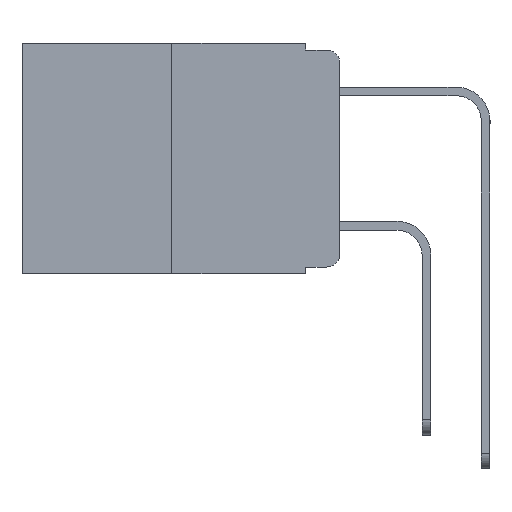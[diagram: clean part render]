
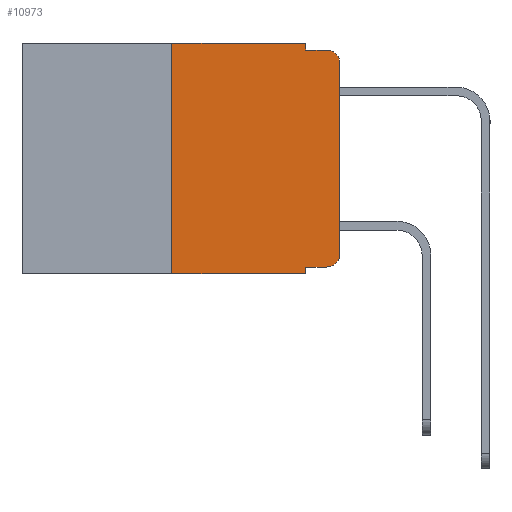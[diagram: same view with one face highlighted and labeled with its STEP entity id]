
A CAD part, left-side view. The second image highlights one B-rep face of the part: STEP entity #10973.
In plain terms, the highlighted planar face has unit normal (-1, 0, 0).
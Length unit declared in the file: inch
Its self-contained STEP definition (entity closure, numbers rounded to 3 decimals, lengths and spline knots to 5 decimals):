
#121 = CARTESIAN_POINT ( 'NONE',  ( 0., 0.25, 0. ) ) ;
#300 = CARTESIAN_POINT ( 'NONE',  ( 0., 0.02, -0.313 ) ) ;
#713 = VECTOR ( 'NONE', #7332, 39.37008 ) ;
#1309 = VECTOR ( 'NONE', #12320, 39.37008 ) ;
#1581 = VERTEX_POINT ( 'NONE', #13843 ) ;
#1685 = CARTESIAN_POINT ( 'NONE',  ( 0., 0.473, -0.343 ) ) ;
#1734 = CARTESIAN_POINT ( 'NONE',  ( 0., 0.473, 0. ) ) ;
#1775 = CARTESIAN_POINT ( 'NONE',  ( 0., 0.051, 0. ) ) ;
#1842 = VECTOR ( 'NONE', #8486, 39.37008 ) ;
#1939 = EDGE_CURVE ( 'NONE', #2662, #12928, #4827, .T. ) ;
#1991 = EDGE_CURVE ( 'NONE', #5677, #5388, #7577, .T. ) ;
#2223 = DIRECTION ( 'NONE',  ( 0., 0., -1. ) ) ;
#2230 = DIRECTION ( 'NONE',  ( -1., 0., 0. ) ) ;
#2281 = VECTOR ( 'NONE', #14022, 39.37008 ) ;
#2423 = AXIS2_PLACEMENT_3D ( 'NONE', #7791, #16998, #9151 ) ;
#2506 = EDGE_CURVE ( 'NONE', #15991, #2662, #7138, .T. ) ;
#2662 = VERTEX_POINT ( 'NONE', #10346 ) ;
#2680 = CARTESIAN_POINT ( 'NONE',  ( 0., 0.051, 0. ) ) ;
#2970 = LINE ( 'NONE', #5135, #10145 ) ;
#3116 = CARTESIAN_POINT ( 'NONE',  ( 0., 0.473, 0. ) ) ;
#3164 = DIRECTION ( 'NONE',  ( 0., 0., -1. ) ) ;
#3512 = ORIENTED_EDGE ( 'NONE', *, *, #13549, .T. ) ;
#4328 = CARTESIAN_POINT ( 'NONE',  ( 0., 0.051, -0.333 ) ) ;
#4356 = EDGE_LOOP ( 'NONE', ( #6258, #3512, #14533, #4379, #8795, #9228, #12717, #9637, #6898, #10875 ) ) ;
#4379 = ORIENTED_EDGE ( 'NONE', *, *, #13575, .F. ) ;
#4827 = LINE ( 'NONE', #7327, #713 ) ;
#4852 = CARTESIAN_POINT ( 'NONE',  ( 0., 0., -0.03 ) ) ;
#4901 = CARTESIAN_POINT ( 'NONE',  ( 0., 0.051, -0.333 ) ) ;
#5135 = CARTESIAN_POINT ( 'NONE',  ( 0., 0.051, 0. ) ) ;
#5388 = VERTEX_POINT ( 'NONE', #12337 ) ;
#5677 = VERTEX_POINT ( 'NONE', #6277 ) ;
#6164 = AXIS2_PLACEMENT_3D ( 'NONE', #1734, #11212, #3164 ) ;
#6258 = ORIENTED_EDGE ( 'NONE', *, *, #1939, .T. ) ;
#6277 = CARTESIAN_POINT ( 'NONE',  ( 0., 0.25, -0.343 ) ) ;
#6898 = ORIENTED_EDGE ( 'NONE', *, *, #10205, .T. ) ;
#6986 = CIRCLE ( 'NONE', #2423, 0.02 ) ;
#7014 = DIRECTION ( 'NONE',  ( 0., 0., 1. ) ) ;
#7138 = CIRCLE ( 'NONE', #13123, 0.02 ) ;
#7327 = CARTESIAN_POINT ( 'NONE',  ( 0., 0., 0. ) ) ;
#7332 = DIRECTION ( 'NONE',  ( 0., 0., 1. ) ) ;
#7577 = LINE ( 'NONE', #121, #10715 ) ;
#7791 = CARTESIAN_POINT ( 'NONE',  ( 0., 0.02, -0.03 ) ) ;
#8486 = DIRECTION ( 'NONE',  ( 0., -1., 0. ) ) ;
#8537 = PLANE ( 'NONE',  #6164 ) ;
#8665 = VERTEX_POINT ( 'NONE', #4901 ) ;
#8795 = ORIENTED_EDGE ( 'NONE', *, *, #13841, .F. ) ;
#9007 = LINE ( 'NONE', #4328, #1309 ) ;
#9151 = DIRECTION ( 'NONE',  ( 0., 0., -1. ) ) ;
#9228 = ORIENTED_EDGE ( 'NONE', *, *, #1991, .F. ) ;
#9637 = ORIENTED_EDGE ( 'NONE', *, *, #9748, .F. ) ;
#9748 = EDGE_CURVE ( 'NONE', #8665, #1581, #10272, .T. ) ;
#10096 = CARTESIAN_POINT ( 'NONE',  ( 0., 0.051, -0.01 ) ) ;
#10145 = VECTOR ( 'NONE', #13110, 39.37008 ) ;
#10205 = EDGE_CURVE ( 'NONE', #8665, #15991, #9007, .T. ) ;
#10272 = LINE ( 'NONE', #1775, #13339 ) ;
#10346 = CARTESIAN_POINT ( 'NONE',  ( 0., 0., -0.313 ) ) ;
#10654 = FACE_OUTER_BOUND ( 'NONE', #4356, .T. ) ;
#10670 = CARTESIAN_POINT ( 'NONE',  ( 0., 0.02, -0.333 ) ) ;
#10715 = VECTOR ( 'NONE', #7014, 39.37008 ) ;
#10875 = ORIENTED_EDGE ( 'NONE', *, *, #2506, .T. ) ;
#10973 = ADVANCED_FACE ( 'NONE', ( #10654 ), #8537, .F. ) ;
#11166 = DIRECTION ( 'NONE',  ( 0., -1., 0. ) ) ;
#11212 = DIRECTION ( 'NONE',  ( 1., 0., 0. ) ) ;
#11922 = VERTEX_POINT ( 'NONE', #2680 ) ;
#12180 = VECTOR ( 'NONE', #11166, 39.37008 ) ;
#12320 = DIRECTION ( 'NONE',  ( 0., -1., 0. ) ) ;
#12337 = CARTESIAN_POINT ( 'NONE',  ( 0., 0.25, 0. ) ) ;
#12591 = LINE ( 'NONE', #3116, #12180 ) ;
#12595 = VERTEX_POINT ( 'NONE', #15995 ) ;
#12717 = ORIENTED_EDGE ( 'NONE', *, *, #13829, .T. ) ;
#12928 = VERTEX_POINT ( 'NONE', #4852 ) ;
#12994 = LINE ( 'NONE', #10096, #2281 ) ;
#13110 = DIRECTION ( 'NONE',  ( 0., 0., -1. ) ) ;
#13123 = AXIS2_PLACEMENT_3D ( 'NONE', #300, #2230, #2223 ) ;
#13339 = VECTOR ( 'NONE', #15181, 39.37008 ) ;
#13549 = EDGE_CURVE ( 'NONE', #12928, #12595, #6986, .T. ) ;
#13575 = EDGE_CURVE ( 'NONE', #11922, #15146, #2970, .T. ) ;
#13829 = EDGE_CURVE ( 'NONE', #5677, #1581, #16059, .T. ) ;
#13841 = EDGE_CURVE ( 'NONE', #5388, #11922, #12591, .T. ) ;
#13843 = CARTESIAN_POINT ( 'NONE',  ( 0., 0.051, -0.343 ) ) ;
#14022 = DIRECTION ( 'NONE',  ( 0., -1., 0. ) ) ;
#14095 = CARTESIAN_POINT ( 'NONE',  ( 0., 0.051, -0.01 ) ) ;
#14533 = ORIENTED_EDGE ( 'NONE', *, *, #15719, .F. ) ;
#15146 = VERTEX_POINT ( 'NONE', #14095 ) ;
#15181 = DIRECTION ( 'NONE',  ( 0., 0., -1. ) ) ;
#15719 = EDGE_CURVE ( 'NONE', #15146, #12595, #12994, .T. ) ;
#15991 = VERTEX_POINT ( 'NONE', #10670 ) ;
#15995 = CARTESIAN_POINT ( 'NONE',  ( 0., 0.02, -0.01 ) ) ;
#16059 = LINE ( 'NONE', #1685, #1842 ) ;
#16998 = DIRECTION ( 'NONE',  ( -1., 0., 0. ) ) ;
